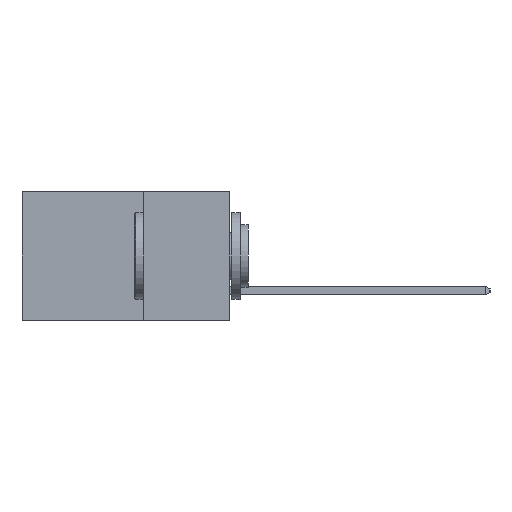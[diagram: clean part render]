
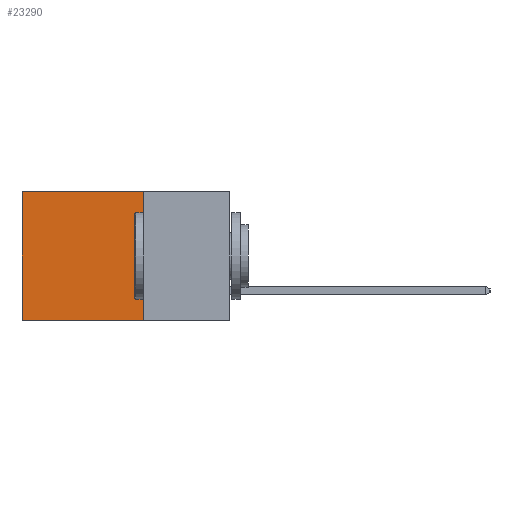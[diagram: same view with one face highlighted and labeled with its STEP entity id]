
A CAD part, left-side view. The second image highlights one B-rep face of the part: STEP entity #23290.
In plain terms, the highlighted planar face has unit normal (-1, 0, 0).
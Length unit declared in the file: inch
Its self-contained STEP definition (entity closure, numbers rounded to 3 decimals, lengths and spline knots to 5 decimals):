
#57 = EDGE_CURVE ( 'NONE', #17463, #16818, #26445, .T. ) ;
#217 = EDGE_CURVE ( 'NONE', #26911, #19238, #10887, .T. ) ;
#2352 = CARTESIAN_POINT ( 'NONE',  ( 0.298, 0.6, -0.37 ) ) ;
#3925 = EDGE_CURVE ( 'NONE', #19238, #16818, #9948, .T. ) ;
#4483 = ORIENTED_EDGE ( 'NONE', *, *, #57, .T. ) ;
#4736 = LINE ( 'NONE', #14358, #19958 ) ;
#5322 = DIRECTION ( 'NONE',  ( 0., 0., -1. ) ) ;
#7332 = CARTESIAN_POINT ( 'NONE',  ( 0.298, 0.25, 0. ) ) ;
#9948 = LINE ( 'NONE', #26410, #25854 ) ;
#10619 = CARTESIAN_POINT ( 'NONE',  ( 0.298, 0.6, 0. ) ) ;
#10808 = EDGE_LOOP ( 'NONE', ( #4483, #13707, #16562, #19508 ) ) ;
#10887 = LINE ( 'NONE', #26055, #26747 ) ;
#12031 = CARTESIAN_POINT ( 'NONE',  ( 0.298, 0.25, -0.37 ) ) ;
#12627 = CARTESIAN_POINT ( 'NONE',  ( 0.298, 0.6, 0. ) ) ;
#13588 = EDGE_CURVE ( 'NONE', #26911, #17463, #4736, .T. ) ;
#13707 = ORIENTED_EDGE ( 'NONE', *, *, #3925, .F. ) ;
#14358 = CARTESIAN_POINT ( 'NONE',  ( 0.298, 0.25, 0. ) ) ;
#14771 = VECTOR ( 'NONE', #23338, 39.37008 ) ;
#15642 = PLANE ( 'NONE',  #17154 ) ;
#16562 = ORIENTED_EDGE ( 'NONE', *, *, #217, .F. ) ;
#16818 = VERTEX_POINT ( 'NONE', #2352 ) ;
#17154 = AXIS2_PLACEMENT_3D ( 'NONE', #7332, #17714, #5322 ) ;
#17463 = VERTEX_POINT ( 'NONE', #10619 ) ;
#17714 = DIRECTION ( 'NONE',  ( 1., 0., 0. ) ) ;
#19238 = VERTEX_POINT ( 'NONE', #12031 ) ;
#19508 = ORIENTED_EDGE ( 'NONE', *, *, #13588, .T. ) ;
#19958 = VECTOR ( 'NONE', #26857, 39.37008 ) ;
#20848 = FACE_OUTER_BOUND ( 'NONE', #10808, .T. ) ;
#22150 = CARTESIAN_POINT ( 'NONE',  ( 0.298, 0.25, 0. ) ) ;
#23290 = ADVANCED_FACE ( 'NONE', ( #20848 ), #15642, .F. ) ;
#23338 = DIRECTION ( 'NONE',  ( 0., 0., -1. ) ) ;
#24159 = DIRECTION ( 'NONE',  ( 0., 0., -1. ) ) ;
#24309 = DIRECTION ( 'NONE',  ( 0., 1., 0. ) ) ;
#25854 = VECTOR ( 'NONE', #24309, 39.37008 ) ;
#26055 = CARTESIAN_POINT ( 'NONE',  ( 0.298, 0.25, 0. ) ) ;
#26410 = CARTESIAN_POINT ( 'NONE',  ( 0.298, 0.25, -0.37 ) ) ;
#26445 = LINE ( 'NONE', #12627, #14771 ) ;
#26747 = VECTOR ( 'NONE', #24159, 39.37008 ) ;
#26857 = DIRECTION ( 'NONE',  ( 0., 1., 0. ) ) ;
#26911 = VERTEX_POINT ( 'NONE', #22150 ) ;
